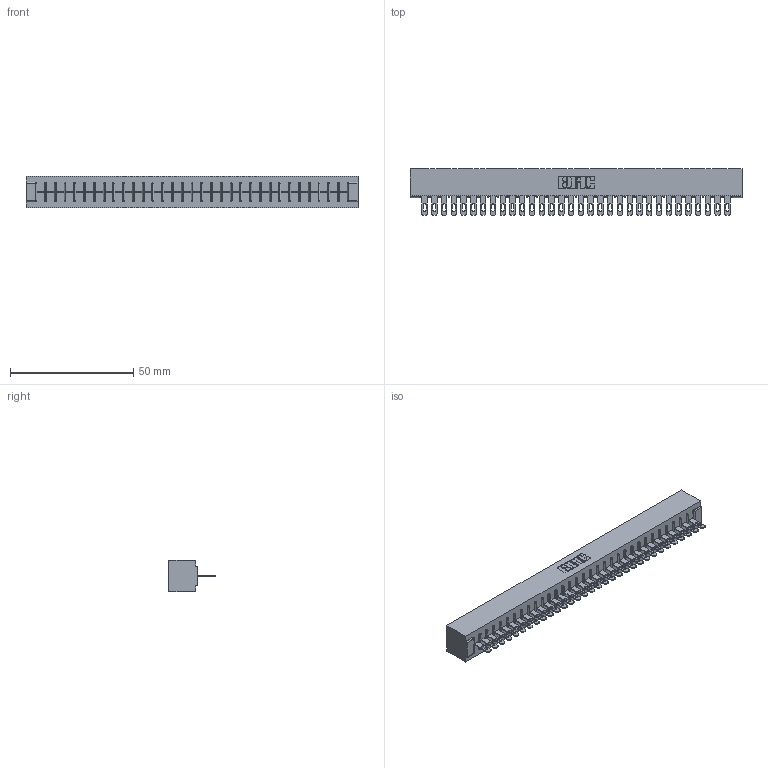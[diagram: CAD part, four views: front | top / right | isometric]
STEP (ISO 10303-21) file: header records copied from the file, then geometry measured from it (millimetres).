
FILE_DESCRIPTION (( 'STEP AP203' ), '1' );
FILE_NAME ('306-032-500-101.STEP', '2019-09-11T22:39:25', ( '' ), ( '' ), 'SwSTEP 2.0', 'SolidWorks 2016', '' );
FILE_SCHEMA (( 'CONFIG_CONTROL_DESIGN' ));
Length unit declared in the file: inch
Products named in the file (3): 306-290-001_100; 306-032-500-101; 306 Part_No Mounting
Assembly tree (33 placements, depth 2):
  306-032-500-101
    306 Part_No Mounting
    306-290-001_100  x32
Bounding box: 134.67 x 18.87 x 12.7 mm (x, y, z)
Volume: 15482 mm3; surface area: 16491.3 mm2
Topology: 33 solids, 33 shells, 2540 faces, 7172 edges, 4608 vertices
Faces by surface type: plane 1664, cylinder 748, sphere 128
Entity records: 31023 total; most frequent: CARTESIAN_POINT 5207, ORIENTED_EDGE 5160, DIRECTION 5136, EDGE_CURVE 2580, VECTOR 2014, LINE 2014, VERTEX_POINT 1632, AXIS2_PLACEMENT_3D 1561
